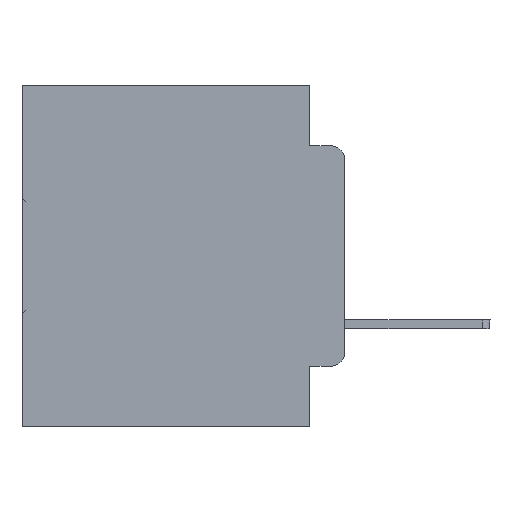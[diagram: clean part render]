
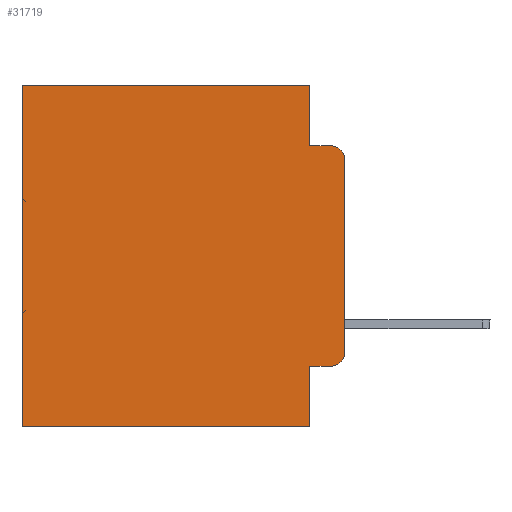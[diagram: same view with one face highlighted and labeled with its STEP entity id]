
A CAD part, left-side view. The second image highlights one B-rep face of the part: STEP entity #31719.
In plain terms, the highlighted planar face has unit normal (-1, 0, 0).
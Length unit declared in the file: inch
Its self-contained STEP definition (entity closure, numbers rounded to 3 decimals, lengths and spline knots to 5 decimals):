
#66 = EDGE_CURVE ( 'NONE', #7206, #17385, #32843, .T. ) ;
#130 = AXIS2_PLACEMENT_3D ( 'NONE', #32325, #18928, #21354 ) ;
#632 = CARTESIAN_POINT ( 'NONE',  ( 0.298, 0.051, -0.0885 ) ) ;
#776 = ORIENTED_EDGE ( 'NONE', *, *, #26891, .T. ) ;
#901 = CARTESIAN_POINT ( 'NONE',  ( 0.298, 0.02, -0.0885 ) ) ;
#2199 = EDGE_CURVE ( 'NONE', #32245, #13742, #8259, .T. ) ;
#2250 = EDGE_CURVE ( 'NONE', #28863, #13742, #26562, .T. ) ;
#2522 = FACE_OUTER_BOUND ( 'NONE', #14297, .T. ) ;
#2829 = CARTESIAN_POINT ( 'NONE',  ( 0.298, 0.051, -0.4115 ) ) ;
#2842 = AXIS2_PLACEMENT_3D ( 'NONE', #4890, #15223, #20675 ) ;
#4890 = CARTESIAN_POINT ( 'NONE',  ( 0.298, 0., 0. ) ) ;
#4929 = DIRECTION ( 'NONE',  ( 0., 0., -1. ) ) ;
#5305 = ORIENTED_EDGE ( 'NONE', *, *, #11530, .F. ) ;
#7013 = VECTOR ( 'NONE', #12293, 39.37008 ) ;
#7206 = VERTEX_POINT ( 'NONE', #2829 ) ;
#7222 = CARTESIAN_POINT ( 'NONE',  ( 0.298, 0.473, 0. ) ) ;
#7245 = CARTESIAN_POINT ( 'NONE',  ( 0.298, 0., -0.3915 ) ) ;
#7283 = ORIENTED_EDGE ( 'NONE', *, *, #2199, .T. ) ;
#7449 = CARTESIAN_POINT ( 'NONE',  ( 0.298, 0., -0.5 ) ) ;
#7750 = DIRECTION ( 'NONE',  ( -1., 0., 0. ) ) ;
#7853 = CARTESIAN_POINT ( 'NONE',  ( 0.298, 0.02, -0.4115 ) ) ;
#8259 = CIRCLE ( 'NONE', #130, 0.02 ) ;
#8904 = ORIENTED_EDGE ( 'NONE', *, *, #66, .T. ) ;
#9537 = VECTOR ( 'NONE', #12332, 39.37008 ) ;
#10320 = PLANE ( 'NONE',  #2842 ) ;
#10355 = CARTESIAN_POINT ( 'NONE',  ( 0.298, 0., 0. ) ) ;
#10509 = CARTESIAN_POINT ( 'NONE',  ( 0.298, 0.473, -0.5 ) ) ;
#10683 = AXIS2_PLACEMENT_3D ( 'NONE', #33341, #7750, #15190 ) ;
#11530 = EDGE_CURVE ( 'NONE', #32065, #31629, #30692, .T. ) ;
#12009 = ORIENTED_EDGE ( 'NONE', *, *, #19157, .F. ) ;
#12291 = CIRCLE ( 'NONE', #10683, 0.02 ) ;
#12293 = DIRECTION ( 'NONE',  ( 0., 1., 0. ) ) ;
#12332 = DIRECTION ( 'NONE',  ( 0., -1., 0. ) ) ;
#12341 = LINE ( 'NONE', #25379, #26161 ) ;
#12845 = DIRECTION ( 'NONE',  ( 0., 0., -1. ) ) ;
#13402 = CARTESIAN_POINT ( 'NONE',  ( 0.298, 0.473, 0. ) ) ;
#13511 = ORIENTED_EDGE ( 'NONE', *, *, #25286, .T. ) ;
#13742 = VERTEX_POINT ( 'NONE', #901 ) ;
#14161 = DIRECTION ( 'NONE',  ( 0., -1., 0. ) ) ;
#14296 = VERTEX_POINT ( 'NONE', #26969 ) ;
#14297 = EDGE_LOOP ( 'NONE', ( #12009, #7283, #29711, #15063, #776, #26813, #5305, #32867, #8904, #13511 ) ) ;
#14315 = CARTESIAN_POINT ( 'NONE',  ( 0.298, 0., 0. ) ) ;
#14850 = VERTEX_POINT ( 'NONE', #7222 ) ;
#15063 = ORIENTED_EDGE ( 'NONE', *, *, #18218, .F. ) ;
#15190 = DIRECTION ( 'NONE',  ( 0., 0., -1. ) ) ;
#15223 = DIRECTION ( 'NONE',  ( 1., 0., 0. ) ) ;
#16719 = CARTESIAN_POINT ( 'NONE',  ( 0.298, 0.051, 0. ) ) ;
#16859 = LINE ( 'NONE', #14315, #7013 ) ;
#17385 = VERTEX_POINT ( 'NONE', #7853 ) ;
#17926 = DIRECTION ( 'NONE',  ( 0., 1., 0. ) ) ;
#17990 = VECTOR ( 'NONE', #14161, 39.37008 ) ;
#18218 = EDGE_CURVE ( 'NONE', #14296, #28863, #12341, .T. ) ;
#18928 = DIRECTION ( 'NONE',  ( -1., 0., 0. ) ) ;
#19154 = LINE ( 'NONE', #13402, #27379 ) ;
#19157 = EDGE_CURVE ( 'NONE', #32245, #32005, #28135, .T. ) ;
#19423 = LINE ( 'NONE', #16719, #20787 ) ;
#20303 = CARTESIAN_POINT ( 'NONE',  ( 0.298, 0.051, -0.5 ) ) ;
#20675 = DIRECTION ( 'NONE',  ( 0., 0., -1. ) ) ;
#20787 = VECTOR ( 'NONE', #29282, 39.37008 ) ;
#20808 = CARTESIAN_POINT ( 'NONE',  ( 0.298, 0., -0.1085 ) ) ;
#21354 = DIRECTION ( 'NONE',  ( 0., 0., -1. ) ) ;
#21822 = EDGE_CURVE ( 'NONE', #7206, #32065, #19423, .T. ) ;
#22436 = VECTOR ( 'NONE', #4929, 39.37008 ) ;
#23994 = VECTOR ( 'NONE', #17926, 39.37008 ) ;
#24386 = CARTESIAN_POINT ( 'NONE',  ( 0.298, 0.051, -0.0885 ) ) ;
#24425 = EDGE_CURVE ( 'NONE', #14850, #31629, #19154, .T. ) ;
#25211 = CARTESIAN_POINT ( 'NONE',  ( 0.298, 0.051, -0.4115 ) ) ;
#25286 = EDGE_CURVE ( 'NONE', #17385, #32005, #12291, .T. ) ;
#25379 = CARTESIAN_POINT ( 'NONE',  ( 0.298, 0.051, 0. ) ) ;
#26161 = VECTOR ( 'NONE', #12845, 39.37008 ) ;
#26562 = LINE ( 'NONE', #632, #17990 ) ;
#26813 = ORIENTED_EDGE ( 'NONE', *, *, #24425, .T. ) ;
#26891 = EDGE_CURVE ( 'NONE', #14296, #14850, #16859, .T. ) ;
#26969 = CARTESIAN_POINT ( 'NONE',  ( 0.298, 0.051, 0. ) ) ;
#27379 = VECTOR ( 'NONE', #29025, 39.37008 ) ;
#28135 = LINE ( 'NONE', #10355, #22436 ) ;
#28863 = VERTEX_POINT ( 'NONE', #24386 ) ;
#29025 = DIRECTION ( 'NONE',  ( 0., 0., -1. ) ) ;
#29282 = DIRECTION ( 'NONE',  ( 0., 0., -1. ) ) ;
#29711 = ORIENTED_EDGE ( 'NONE', *, *, #2250, .F. ) ;
#30692 = LINE ( 'NONE', #7449, #23994 ) ;
#31629 = VERTEX_POINT ( 'NONE', #10509 ) ;
#31719 = ADVANCED_FACE ( 'NONE', ( #2522 ), #10320, .F. ) ;
#32005 = VERTEX_POINT ( 'NONE', #7245 ) ;
#32065 = VERTEX_POINT ( 'NONE', #20303 ) ;
#32245 = VERTEX_POINT ( 'NONE', #20808 ) ;
#32325 = CARTESIAN_POINT ( 'NONE',  ( 0.298, 0.02, -0.1085 ) ) ;
#32843 = LINE ( 'NONE', #25211, #9537 ) ;
#32867 = ORIENTED_EDGE ( 'NONE', *, *, #21822, .F. ) ;
#33341 = CARTESIAN_POINT ( 'NONE',  ( 0.298, 0.02, -0.3915 ) ) ;
